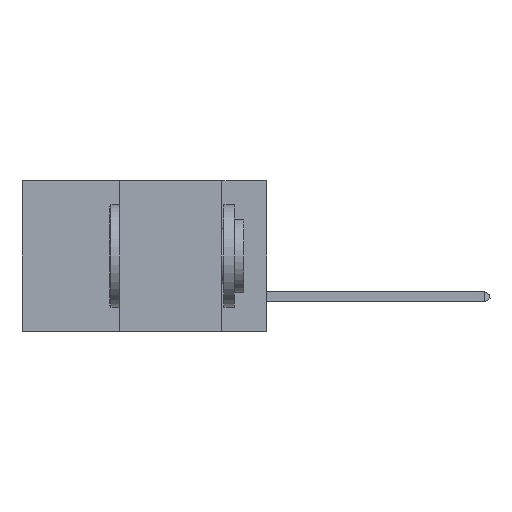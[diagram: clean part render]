
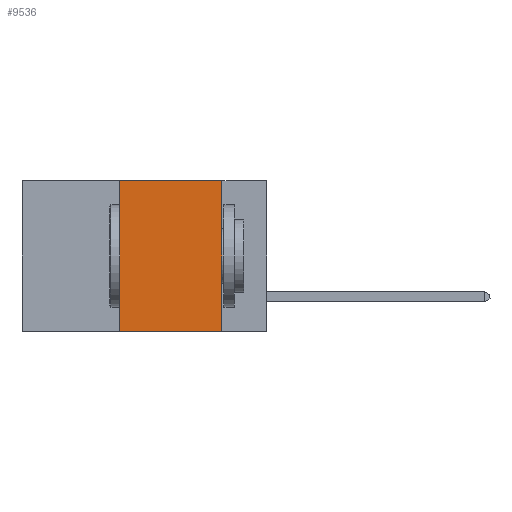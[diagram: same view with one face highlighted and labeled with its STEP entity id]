
A CAD part, left-side view. The second image highlights one B-rep face of the part: STEP entity #9536.
In plain terms, the highlighted planar face has unit normal (-1, 0, 0).
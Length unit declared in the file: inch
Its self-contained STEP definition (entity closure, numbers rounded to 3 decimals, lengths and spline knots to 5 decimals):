
#504 = VERTEX_POINT ( 'NONE', #5657 ) ;
#1053 = DIRECTION ( 'NONE',  ( 0., 0., -1. ) ) ;
#1173 = CARTESIAN_POINT ( 'NONE',  ( 0., 0.11, 0. ) ) ;
#1656 = CARTESIAN_POINT ( 'NONE',  ( 0., 0.6, 0. ) ) ;
#2565 = VECTOR ( 'NONE', #12885, 39.37008 ) ;
#2693 = PLANE ( 'NONE',  #10783 ) ;
#3118 = VECTOR ( 'NONE', #1053, 39.37008 ) ;
#3703 = CARTESIAN_POINT ( 'NONE',  ( 0., 0.6, 0. ) ) ;
#3960 = EDGE_CURVE ( 'NONE', #11923, #504, #10639, .T. ) ;
#4688 = CARTESIAN_POINT ( 'NONE',  ( 0., 0.11, 0. ) ) ;
#4734 = CARTESIAN_POINT ( 'NONE',  ( 0., 0.6, -0.37 ) ) ;
#4799 = DIRECTION ( 'NONE',  ( 1., 0., 0. ) ) ;
#5514 = ORIENTED_EDGE ( 'NONE', *, *, #6835, .F. ) ;
#5642 = ORIENTED_EDGE ( 'NONE', *, *, #11574, .F. ) ;
#5657 = CARTESIAN_POINT ( 'NONE',  ( 0., 0.36, 0. ) ) ;
#5998 = LINE ( 'NONE', #1173, #3118 ) ;
#6434 = VERTEX_POINT ( 'NONE', #4688 ) ;
#6714 = ORIENTED_EDGE ( 'NONE', *, *, #3960, .F. ) ;
#6835 = EDGE_CURVE ( 'NONE', #6434, #7113, #5998, .T. ) ;
#7075 = ORIENTED_EDGE ( 'NONE', *, *, #8151, .T. ) ;
#7113 = VERTEX_POINT ( 'NONE', #9973 ) ;
#8151 = EDGE_CURVE ( 'NONE', #11923, #7113, #12104, .T. ) ;
#8285 = CARTESIAN_POINT ( 'NONE',  ( 0., 0.36, -0.37 ) ) ;
#9506 = FACE_OUTER_BOUND ( 'NONE', #11583, .T. ) ;
#9536 = ADVANCED_FACE ( 'NONE', ( #9506 ), #2693, .F. ) ;
#9594 = VECTOR ( 'NONE', #10736, 39.37008 ) ;
#9772 = VECTOR ( 'NONE', #11749, 39.37008 ) ;
#9973 = CARTESIAN_POINT ( 'NONE',  ( 0., 0.11, -0.37 ) ) ;
#10639 = LINE ( 'NONE', #12816, #2565 ) ;
#10736 = DIRECTION ( 'NONE',  ( 0., -1., 0. ) ) ;
#10783 = AXIS2_PLACEMENT_3D ( 'NONE', #3703, #4799, #11800 ) ;
#11574 = EDGE_CURVE ( 'NONE', #504, #6434, #12227, .T. ) ;
#11583 = EDGE_LOOP ( 'NONE', ( #5514, #5642, #6714, #7075 ) ) ;
#11749 = DIRECTION ( 'NONE',  ( 0., -1., 0. ) ) ;
#11800 = DIRECTION ( 'NONE',  ( 0., 0., -1. ) ) ;
#11923 = VERTEX_POINT ( 'NONE', #8285 ) ;
#12104 = LINE ( 'NONE', #4734, #9772 ) ;
#12227 = LINE ( 'NONE', #1656, #9594 ) ;
#12816 = CARTESIAN_POINT ( 'NONE',  ( 0., 0.36, 0. ) ) ;
#12885 = DIRECTION ( 'NONE',  ( 0., 0., 1. ) ) ;
